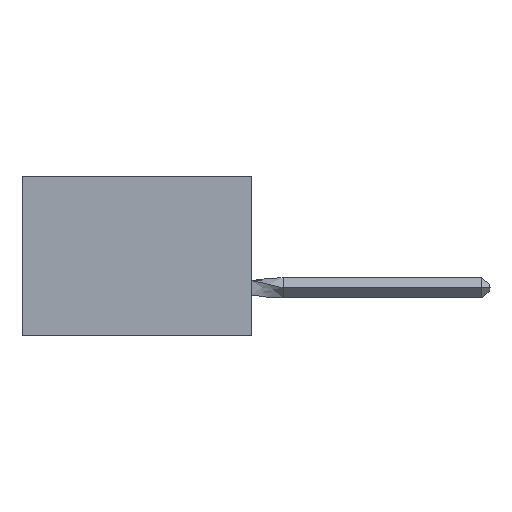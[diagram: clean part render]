
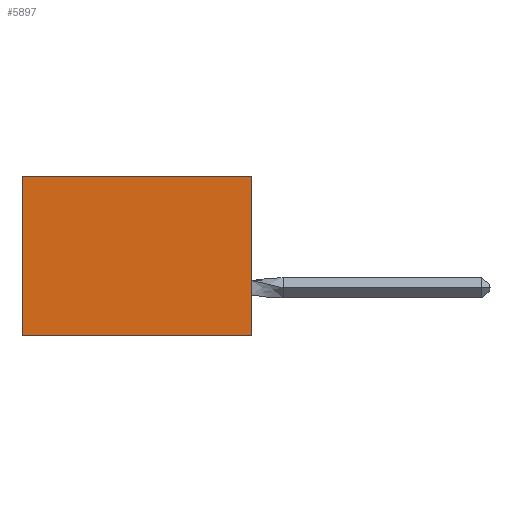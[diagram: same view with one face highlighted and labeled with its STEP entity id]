
A CAD part, left-side view. The second image highlights one B-rep face of the part: STEP entity #5897.
In plain terms, the highlighted planar face has unit normal (-1, 0, 0).
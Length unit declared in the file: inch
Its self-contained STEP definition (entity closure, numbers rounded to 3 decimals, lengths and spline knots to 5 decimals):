
#341 = DIRECTION ( 'NONE',  ( 0., 1., 0. ) ) ;
#1356 = LINE ( 'NONE', #9464, #8437 ) ;
#1366 = DIRECTION ( 'NONE',  ( 0., 0., -1. ) ) ;
#1876 = ORIENTED_EDGE ( 'NONE', *, *, #16940, .T. ) ;
#2106 = CARTESIAN_POINT ( 'NONE',  ( 0.305, 0., -0.5 ) ) ;
#2116 = CARTESIAN_POINT ( 'NONE',  ( 0.305, 0., -0.5 ) ) ;
#2347 = CARTESIAN_POINT ( 'NONE',  ( 0.305, 0.72, -0.5 ) ) ;
#2420 = ORIENTED_EDGE ( 'NONE', *, *, #5128, .T. ) ;
#2504 = CARTESIAN_POINT ( 'NONE',  ( 0.305, 0., -0.5 ) ) ;
#3915 = EDGE_CURVE ( 'NONE', #8420, #4954, #12395, .T. ) ;
#4954 = VERTEX_POINT ( 'NONE', #6734 ) ;
#5094 = FACE_OUTER_BOUND ( 'NONE', #13581, .T. ) ;
#5128 = EDGE_CURVE ( 'NONE', #8420, #16428, #1356, .T. ) ;
#5660 = EDGE_CURVE ( 'NONE', #4954, #11641, #10502, .T. ) ;
#5717 = DIRECTION ( 'NONE',  ( 0., 0., -1. ) ) ;
#5897 = ADVANCED_FACE ( 'NONE', ( #5094 ), #9256, .F. ) ;
#6186 = DIRECTION ( 'NONE',  ( 0., 0., -1. ) ) ;
#6734 = CARTESIAN_POINT ( 'NONE',  ( 0.305, 0., -0.5 ) ) ;
#7101 = CARTESIAN_POINT ( 'NONE',  ( 0.305, 0.72, -0.5 ) ) ;
#8420 = VERTEX_POINT ( 'NONE', #16457 ) ;
#8437 = VECTOR ( 'NONE', #341, 39.37008 ) ;
#9256 = PLANE ( 'NONE',  #12412 ) ;
#9366 = ORIENTED_EDGE ( 'NONE', *, *, #3915, .F. ) ;
#9464 = CARTESIAN_POINT ( 'NONE',  ( 0.305, 0., 0. ) ) ;
#10502 = LINE ( 'NONE', #2116, #13595 ) ;
#10582 = DIRECTION ( 'NONE',  ( 1., 0., 0. ) ) ;
#11343 = ORIENTED_EDGE ( 'NONE', *, *, #5660, .F. ) ;
#11404 = DIRECTION ( 'NONE',  ( 0., 1., 0. ) ) ;
#11641 = VERTEX_POINT ( 'NONE', #2347 ) ;
#12236 = VECTOR ( 'NONE', #5717, 39.37008 ) ;
#12395 = LINE ( 'NONE', #2106, #12796 ) ;
#12412 = AXIS2_PLACEMENT_3D ( 'NONE', #2504, #10582, #1366 ) ;
#12796 = VECTOR ( 'NONE', #6186, 39.37008 ) ;
#12837 = LINE ( 'NONE', #7101, #12236 ) ;
#13581 = EDGE_LOOP ( 'NONE', ( #1876, #11343, #9366, #2420 ) ) ;
#13595 = VECTOR ( 'NONE', #11404, 39.37008 ) ;
#15222 = CARTESIAN_POINT ( 'NONE',  ( 0.305, 0.72, 0. ) ) ;
#16428 = VERTEX_POINT ( 'NONE', #15222 ) ;
#16457 = CARTESIAN_POINT ( 'NONE',  ( 0.305, 0., 0. ) ) ;
#16940 = EDGE_CURVE ( 'NONE', #16428, #11641, #12837, .T. ) ;
